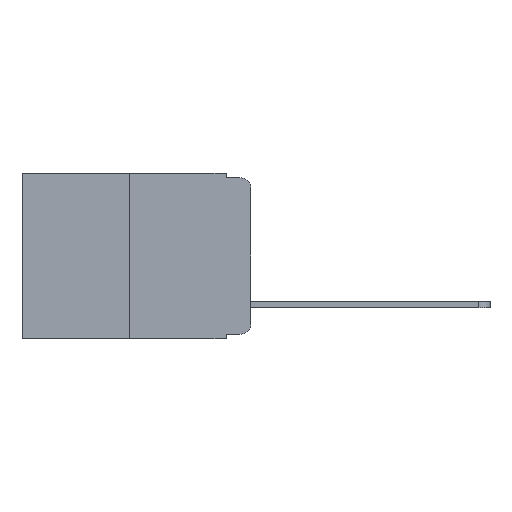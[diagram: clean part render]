
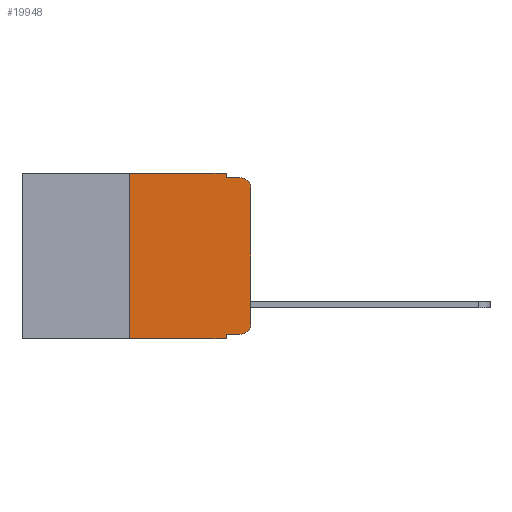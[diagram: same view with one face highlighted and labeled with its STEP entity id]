
A CAD part, left-side view. The second image highlights one B-rep face of the part: STEP entity #19948.
In plain terms, the highlighted planar face has unit normal (-1, 0, 0).
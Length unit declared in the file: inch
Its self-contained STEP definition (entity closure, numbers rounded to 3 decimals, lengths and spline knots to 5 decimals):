
#1000 = CARTESIAN_POINT ( 'NONE',  ( 0., 0.051, -0.333 ) ) ;
#1073 = FACE_OUTER_BOUND ( 'NONE', #8165, .T. ) ;
#1380 = LINE ( 'NONE', #11329, #10499 ) ;
#2092 = EDGE_CURVE ( 'NONE', #3507, #10277, #5128, .T. ) ;
#2096 = DIRECTION ( 'NONE',  ( 0., 0., -1. ) ) ;
#2493 = VERTEX_POINT ( 'NONE', #12340 ) ;
#2759 = EDGE_CURVE ( 'NONE', #14672, #12299, #4240, .T. ) ;
#3006 = LINE ( 'NONE', #14833, #16006 ) ;
#3100 = VERTEX_POINT ( 'NONE', #17448 ) ;
#3156 = ORIENTED_EDGE ( 'NONE', *, *, #18965, .F. ) ;
#3165 = CARTESIAN_POINT ( 'NONE',  ( 0., 0.02, -0.01 ) ) ;
#3507 = VERTEX_POINT ( 'NONE', #9806 ) ;
#4240 = CIRCLE ( 'NONE', #12738, 0.02 ) ;
#4432 = LINE ( 'NONE', #1000, #9223 ) ;
#5125 = VERTEX_POINT ( 'NONE', #16175 ) ;
#5128 = LINE ( 'NONE', #18144, #10368 ) ;
#5436 = LINE ( 'NONE', #6310, #18015 ) ;
#5447 = ORIENTED_EDGE ( 'NONE', *, *, #14438, .T. ) ;
#5725 = VERTEX_POINT ( 'NONE', #19891 ) ;
#5893 = EDGE_CURVE ( 'NONE', #5725, #3100, #20248, .T. ) ;
#6066 = ORIENTED_EDGE ( 'NONE', *, *, #10048, .F. ) ;
#6310 = CARTESIAN_POINT ( 'NONE',  ( 0., 0.473, 0. ) ) ;
#6588 = ORIENTED_EDGE ( 'NONE', *, *, #5893, .F. ) ;
#7003 = VECTOR ( 'NONE', #14860, 39.37008 ) ;
#7193 = CARTESIAN_POINT ( 'NONE',  ( 0., 0., -0.313 ) ) ;
#7525 = DIRECTION ( 'NONE',  ( 0., 0., -1. ) ) ;
#7637 = PLANE ( 'NONE',  #13871 ) ;
#8032 = DIRECTION ( 'NONE',  ( 0., 0., -1. ) ) ;
#8165 = EDGE_LOOP ( 'NONE', ( #5447, #17790, #3156, #17088, #6066, #6588, #13673, #18289, #8572, #13439 ) ) ;
#8233 = CARTESIAN_POINT ( 'NONE',  ( 0., 0.02, -0.313 ) ) ;
#8572 = ORIENTED_EDGE ( 'NONE', *, *, #19521, .T. ) ;
#9000 = VERTEX_POINT ( 'NONE', #7193 ) ;
#9223 = VECTOR ( 'NONE', #13381, 39.37008 ) ;
#9411 = DIRECTION ( 'NONE',  ( 0., 0., -1. ) ) ;
#9806 = CARTESIAN_POINT ( 'NONE',  ( 0., 0.051, -0.333 ) ) ;
#9970 = DIRECTION ( 'NONE',  ( 0., 0., -1. ) ) ;
#10048 = EDGE_CURVE ( 'NONE', #3100, #5125, #5436, .T. ) ;
#10277 = VERTEX_POINT ( 'NONE', #16703 ) ;
#10368 = VECTOR ( 'NONE', #7525, 39.37008 ) ;
#10499 = VECTOR ( 'NONE', #12935, 39.37008 ) ;
#10606 = AXIS2_PLACEMENT_3D ( 'NONE', #8233, #19368, #9970 ) ;
#11329 = CARTESIAN_POINT ( 'NONE',  ( 0., 0.473, -0.343 ) ) ;
#11331 = CIRCLE ( 'NONE', #10606, 0.02 ) ;
#12015 = VECTOR ( 'NONE', #2096, 39.37008 ) ;
#12272 = CARTESIAN_POINT ( 'NONE',  ( 0., 0.051, -0.01 ) ) ;
#12299 = VERTEX_POINT ( 'NONE', #3165 ) ;
#12340 = CARTESIAN_POINT ( 'NONE',  ( 0., 0.02, -0.333 ) ) ;
#12738 = AXIS2_PLACEMENT_3D ( 'NONE', #20668, #19201, #8032 ) ;
#12935 = DIRECTION ( 'NONE',  ( 0., -1., 0. ) ) ;
#13261 = DIRECTION ( 'NONE',  ( 0., -1., 0. ) ) ;
#13286 = CARTESIAN_POINT ( 'NONE',  ( 0., 0., 0. ) ) ;
#13381 = DIRECTION ( 'NONE',  ( 0., -1., 0. ) ) ;
#13439 = ORIENTED_EDGE ( 'NONE', *, *, #13757, .T. ) ;
#13673 = ORIENTED_EDGE ( 'NONE', *, *, #14911, .T. ) ;
#13757 = EDGE_CURVE ( 'NONE', #2493, #9000, #11331, .T. ) ;
#13871 = AXIS2_PLACEMENT_3D ( 'NONE', #18729, #18862, #9411 ) ;
#14377 = DIRECTION ( 'NONE',  ( 0., 0., 1. ) ) ;
#14438 = EDGE_CURVE ( 'NONE', #9000, #14672, #19793, .T. ) ;
#14672 = VERTEX_POINT ( 'NONE', #21441 ) ;
#14820 = EDGE_CURVE ( 'NONE', #5125, #19760, #16687, .T. ) ;
#14833 = CARTESIAN_POINT ( 'NONE',  ( 0., 0.051, -0.01 ) ) ;
#14860 = DIRECTION ( 'NONE',  ( 0., 0., 1. ) ) ;
#14911 = EDGE_CURVE ( 'NONE', #5725, #10277, #1380, .T. ) ;
#16006 = VECTOR ( 'NONE', #13261, 39.37008 ) ;
#16175 = CARTESIAN_POINT ( 'NONE',  ( 0., 0.051, 0. ) ) ;
#16199 = VECTOR ( 'NONE', #14377, 39.37008 ) ;
#16687 = LINE ( 'NONE', #17367, #12015 ) ;
#16703 = CARTESIAN_POINT ( 'NONE',  ( 0., 0.051, -0.343 ) ) ;
#17088 = ORIENTED_EDGE ( 'NONE', *, *, #14820, .F. ) ;
#17367 = CARTESIAN_POINT ( 'NONE',  ( 0., 0.051, 0. ) ) ;
#17448 = CARTESIAN_POINT ( 'NONE',  ( 0., 0.25, 0. ) ) ;
#17727 = DIRECTION ( 'NONE',  ( 0., -1., 0. ) ) ;
#17790 = ORIENTED_EDGE ( 'NONE', *, *, #2759, .T. ) ;
#18015 = VECTOR ( 'NONE', #17727, 39.37008 ) ;
#18144 = CARTESIAN_POINT ( 'NONE',  ( 0., 0.051, 0. ) ) ;
#18289 = ORIENTED_EDGE ( 'NONE', *, *, #2092, .F. ) ;
#18729 = CARTESIAN_POINT ( 'NONE',  ( 0., 0.473, 0. ) ) ;
#18862 = DIRECTION ( 'NONE',  ( 1., 0., 0. ) ) ;
#18965 = EDGE_CURVE ( 'NONE', #19760, #12299, #3006, .T. ) ;
#19201 = DIRECTION ( 'NONE',  ( -1., 0., 0. ) ) ;
#19368 = DIRECTION ( 'NONE',  ( -1., 0., 0. ) ) ;
#19521 = EDGE_CURVE ( 'NONE', #3507, #2493, #4432, .T. ) ;
#19760 = VERTEX_POINT ( 'NONE', #12272 ) ;
#19793 = LINE ( 'NONE', #13286, #7003 ) ;
#19891 = CARTESIAN_POINT ( 'NONE',  ( 0., 0.25, -0.343 ) ) ;
#19948 = ADVANCED_FACE ( 'NONE', ( #1073 ), #7637, .F. ) ;
#20248 = LINE ( 'NONE', #20465, #16199 ) ;
#20465 = CARTESIAN_POINT ( 'NONE',  ( 0., 0.25, 0. ) ) ;
#20668 = CARTESIAN_POINT ( 'NONE',  ( 0., 0.02, -0.03 ) ) ;
#21441 = CARTESIAN_POINT ( 'NONE',  ( 0., 0., -0.03 ) ) ;
